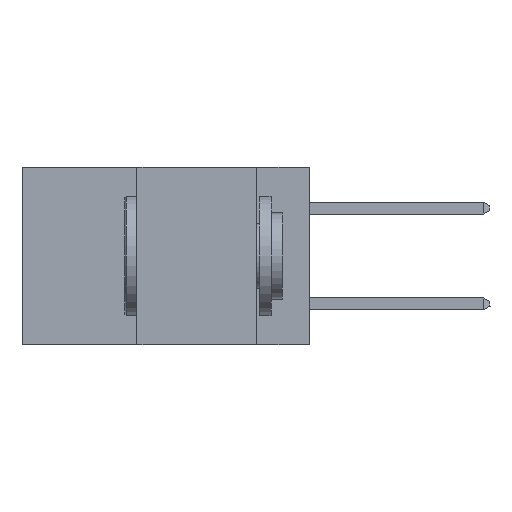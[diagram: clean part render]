
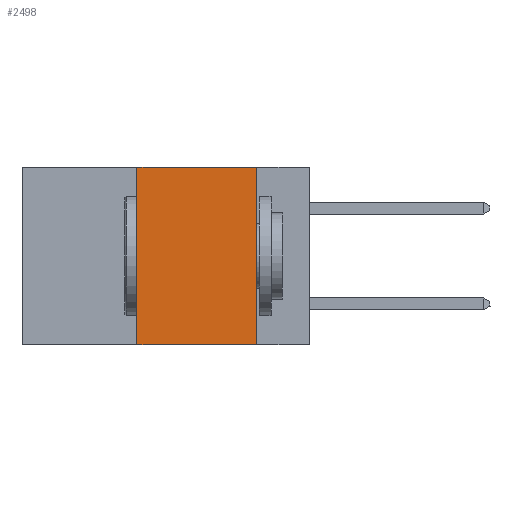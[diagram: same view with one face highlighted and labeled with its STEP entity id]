
A CAD part, left-side view. The second image highlights one B-rep face of the part: STEP entity #2498.
In plain terms, the highlighted planar face has unit normal (-1, 0, 0).
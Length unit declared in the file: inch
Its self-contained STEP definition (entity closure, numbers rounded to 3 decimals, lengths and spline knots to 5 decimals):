
#333 = ORIENTED_EDGE ( 'NONE', *, *, #12024, .F. ) ;
#1261 = VECTOR ( 'NONE', #11404, 39.37008 ) ;
#1534 = CARTESIAN_POINT ( 'NONE',  ( 0., 0.36, -0.37 ) ) ;
#1843 = EDGE_CURVE ( 'NONE', #8432, #15993, #12854, .T. ) ;
#2231 = DIRECTION ( 'NONE',  ( 0., 0., 1. ) ) ;
#2345 = DIRECTION ( 'NONE',  ( 0., 0., -1. ) ) ;
#2498 = ADVANCED_FACE ( 'NONE', ( #13760 ), #4962, .F. ) ;
#2947 = EDGE_LOOP ( 'NONE', ( #9378, #12966, #333, #4628 ) ) ;
#3631 = DIRECTION ( 'NONE',  ( 0., 0., -1. ) ) ;
#3647 = VECTOR ( 'NONE', #2345, 39.37008 ) ;
#4628 = ORIENTED_EDGE ( 'NONE', *, *, #8230, .T. ) ;
#4962 = PLANE ( 'NONE',  #11194 ) ;
#5648 = VECTOR ( 'NONE', #13087, 39.37008 ) ;
#5835 = CARTESIAN_POINT ( 'NONE',  ( 0., 0.11, 0. ) ) ;
#7374 = EDGE_CURVE ( 'NONE', #15993, #13431, #15314, .T. ) ;
#7584 = VECTOR ( 'NONE', #2231, 39.37008 ) ;
#8230 = EDGE_CURVE ( 'NONE', #13725, #13431, #11934, .T. ) ;
#8432 = VERTEX_POINT ( 'NONE', #17414 ) ;
#9378 = ORIENTED_EDGE ( 'NONE', *, *, #7374, .F. ) ;
#10419 = CARTESIAN_POINT ( 'NONE',  ( 0., 0.11, 0. ) ) ;
#10892 = LINE ( 'NONE', #13306, #7584 ) ;
#11194 = AXIS2_PLACEMENT_3D ( 'NONE', #12127, #16438, #3631 ) ;
#11404 = DIRECTION ( 'NONE',  ( 0., -1., 0. ) ) ;
#11934 = LINE ( 'NONE', #15423, #1261 ) ;
#12024 = EDGE_CURVE ( 'NONE', #13725, #8432, #10892, .T. ) ;
#12127 = CARTESIAN_POINT ( 'NONE',  ( 0., 0.6, 0. ) ) ;
#12854 = LINE ( 'NONE', #17432, #5648 ) ;
#12966 = ORIENTED_EDGE ( 'NONE', *, *, #1843, .F. ) ;
#13087 = DIRECTION ( 'NONE',  ( 0., -1., 0. ) ) ;
#13306 = CARTESIAN_POINT ( 'NONE',  ( 0., 0.36, 0. ) ) ;
#13431 = VERTEX_POINT ( 'NONE', #15741 ) ;
#13725 = VERTEX_POINT ( 'NONE', #1534 ) ;
#13760 = FACE_OUTER_BOUND ( 'NONE', #2947, .T. ) ;
#15314 = LINE ( 'NONE', #5835, #3647 ) ;
#15423 = CARTESIAN_POINT ( 'NONE',  ( 0., 0.6, -0.37 ) ) ;
#15741 = CARTESIAN_POINT ( 'NONE',  ( 0., 0.11, -0.37 ) ) ;
#15993 = VERTEX_POINT ( 'NONE', #10419 ) ;
#16438 = DIRECTION ( 'NONE',  ( 1., 0., 0. ) ) ;
#17414 = CARTESIAN_POINT ( 'NONE',  ( 0., 0.36, 0. ) ) ;
#17432 = CARTESIAN_POINT ( 'NONE',  ( 0., 0.6, 0. ) ) ;
